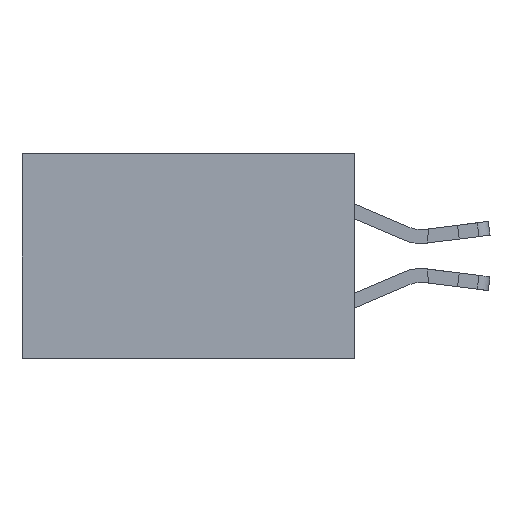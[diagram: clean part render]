
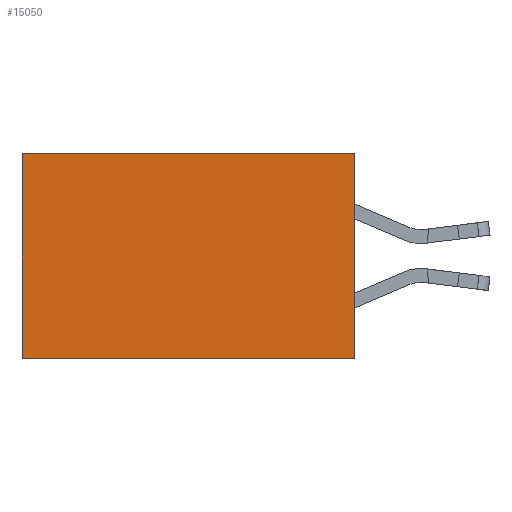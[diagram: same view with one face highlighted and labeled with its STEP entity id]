
A CAD part, left-side view. The second image highlights one B-rep face of the part: STEP entity #15050.
In plain terms, the highlighted planar face has unit normal (-1, 0, 0).
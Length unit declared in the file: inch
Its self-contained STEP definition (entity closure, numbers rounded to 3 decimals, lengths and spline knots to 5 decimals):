
#114 = DIRECTION ( 'NONE',  ( 0., 0., -1. ) ) ;
#597 = DIRECTION ( 'NONE',  ( 1., 0., 0. ) ) ;
#1005 = CARTESIAN_POINT ( 'NONE',  ( 0.2615, 0.6, -0.37 ) ) ;
#1319 = LINE ( 'NONE', #5811, #12210 ) ;
#1762 = CARTESIAN_POINT ( 'NONE',  ( 0.2615, 0., -0.37 ) ) ;
#1861 = ORIENTED_EDGE ( 'NONE', *, *, #14335, .T. ) ;
#1884 = EDGE_CURVE ( 'NONE', #13123, #13349, #1319, .T. ) ;
#1991 = PLANE ( 'NONE',  #9266 ) ;
#2353 = DIRECTION ( 'NONE',  ( 0., 1., 0. ) ) ;
#2760 = EDGE_CURVE ( 'NONE', #7275, #8653, #3744, .T. ) ;
#2821 = DIRECTION ( 'NONE',  ( 0., 1., 0. ) ) ;
#2887 = ORIENTED_EDGE ( 'NONE', *, *, #4976, .F. ) ;
#3001 = DIRECTION ( 'NONE',  ( 0., 0., -1. ) ) ;
#3287 = LINE ( 'NONE', #12872, #8257 ) ;
#3376 = LINE ( 'NONE', #10494, #12111 ) ;
#3744 = LINE ( 'NONE', #7294, #13064 ) ;
#4976 = EDGE_CURVE ( 'NONE', #13349, #8653, #3376, .T. ) ;
#5596 = EDGE_LOOP ( 'NONE', ( #7055, #2887, #14120, #1861 ) ) ;
#5811 = CARTESIAN_POINT ( 'NONE',  ( 0.2615, 0., -0.37 ) ) ;
#7055 = ORIENTED_EDGE ( 'NONE', *, *, #2760, .T. ) ;
#7275 = VERTEX_POINT ( 'NONE', #8015 ) ;
#7294 = CARTESIAN_POINT ( 'NONE',  ( 0.2615, 0.6, -0.37 ) ) ;
#8015 = CARTESIAN_POINT ( 'NONE',  ( 0.2615, 0.6, 0. ) ) ;
#8257 = VECTOR ( 'NONE', #2353, 39.37008 ) ;
#8653 = VERTEX_POINT ( 'NONE', #1005 ) ;
#8905 = CARTESIAN_POINT ( 'NONE',  ( 0.2615, 0., -0.37 ) ) ;
#9035 = FACE_OUTER_BOUND ( 'NONE', #5596, .T. ) ;
#9266 = AXIS2_PLACEMENT_3D ( 'NONE', #1762, #597, #3001 ) ;
#10494 = CARTESIAN_POINT ( 'NONE',  ( 0.2615, 0., -0.37 ) ) ;
#11925 = DIRECTION ( 'NONE',  ( 0., 0., -1. ) ) ;
#12111 = VECTOR ( 'NONE', #2821, 39.37008 ) ;
#12210 = VECTOR ( 'NONE', #11925, 39.37008 ) ;
#12643 = CARTESIAN_POINT ( 'NONE',  ( 0.2615, 0., 0. ) ) ;
#12872 = CARTESIAN_POINT ( 'NONE',  ( 0.2615, 0., 0. ) ) ;
#13064 = VECTOR ( 'NONE', #114, 39.37008 ) ;
#13123 = VERTEX_POINT ( 'NONE', #12643 ) ;
#13349 = VERTEX_POINT ( 'NONE', #8905 ) ;
#14120 = ORIENTED_EDGE ( 'NONE', *, *, #1884, .F. ) ;
#14335 = EDGE_CURVE ( 'NONE', #13123, #7275, #3287, .T. ) ;
#15050 = ADVANCED_FACE ( 'NONE', ( #9035 ), #1991, .F. ) ;
